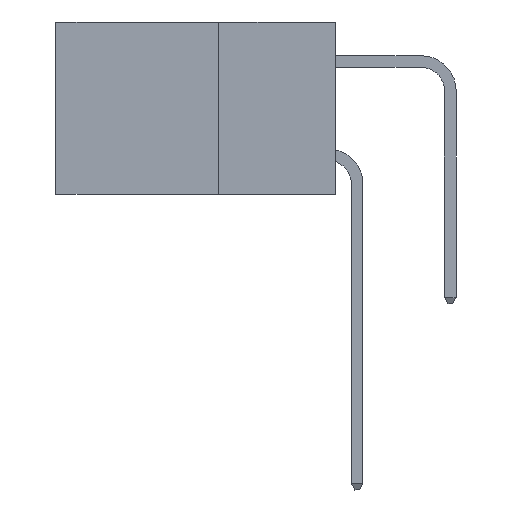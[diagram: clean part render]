
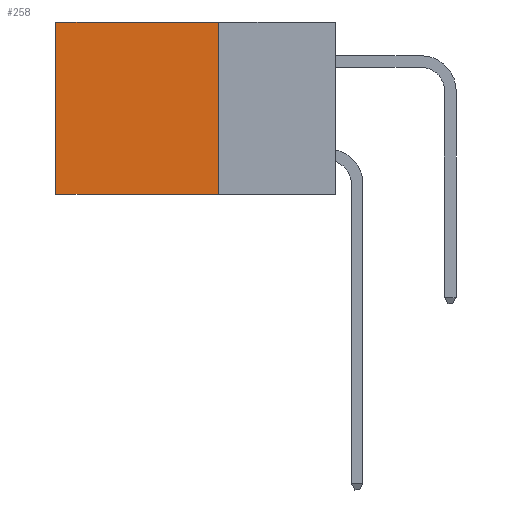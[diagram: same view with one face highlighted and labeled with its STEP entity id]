
A CAD part, left-side view. The second image highlights one B-rep face of the part: STEP entity #258.
In plain terms, the highlighted planar face has unit normal (-1, 0, 0).
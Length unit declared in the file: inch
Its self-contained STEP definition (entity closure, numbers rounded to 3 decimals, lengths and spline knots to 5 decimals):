
#137 = EDGE_CURVE ( 'NONE', #5215, #2214, #8171, .T. ) ;
#258 = ADVANCED_FACE ( 'NONE', ( #6620 ), #11562, .F. ) ;
#606 = DIRECTION ( 'NONE',  ( 0., 0., -1. ) ) ;
#1831 = CARTESIAN_POINT ( 'NONE',  ( 0.2875, 0.25, -0.37 ) ) ;
#1930 = DIRECTION ( 'NONE',  ( 0., 0., -1. ) ) ;
#1971 = CARTESIAN_POINT ( 'NONE',  ( 0.2875, 0.25, 0. ) ) ;
#2177 = LINE ( 'NONE', #2219, #7126 ) ;
#2214 = VERTEX_POINT ( 'NONE', #7448 ) ;
#2219 = CARTESIAN_POINT ( 'NONE',  ( 0.2875, 0.6, 0. ) ) ;
#3072 = VERTEX_POINT ( 'NONE', #8707 ) ;
#3559 = LINE ( 'NONE', #8544, #8493 ) ;
#3839 = CARTESIAN_POINT ( 'NONE',  ( 0.2875, 0.25, -0.37 ) ) ;
#4750 = CARTESIAN_POINT ( 'NONE',  ( 0.2875, 0.25, 0. ) ) ;
#5052 = EDGE_CURVE ( 'NONE', #3072, #2214, #2177, .T. ) ;
#5160 = DIRECTION ( 'NONE',  ( 1., 0., 0. ) ) ;
#5215 = VERTEX_POINT ( 'NONE', #3839 ) ;
#5244 = DIRECTION ( 'NONE',  ( 0., 0., -1. ) ) ;
#5316 = DIRECTION ( 'NONE',  ( 0., 1., 0. ) ) ;
#5541 = VECTOR ( 'NONE', #5316, 39.37008 ) ;
#5803 = AXIS2_PLACEMENT_3D ( 'NONE', #4750, #5160, #5244 ) ;
#5904 = ORIENTED_EDGE ( 'NONE', *, *, #5052, .T. ) ;
#6285 = VECTOR ( 'NONE', #11564, 39.37008 ) ;
#6306 = EDGE_CURVE ( 'NONE', #7110, #5215, #3559, .T. ) ;
#6620 = FACE_OUTER_BOUND ( 'NONE', #10270, .T. ) ;
#6824 = ORIENTED_EDGE ( 'NONE', *, *, #137, .F. ) ;
#7110 = VERTEX_POINT ( 'NONE', #10471 ) ;
#7126 = VECTOR ( 'NONE', #1930, 39.37008 ) ;
#7435 = ORIENTED_EDGE ( 'NONE', *, *, #6306, .F. ) ;
#7448 = CARTESIAN_POINT ( 'NONE',  ( 0.2875, 0.6, -0.37 ) ) ;
#7653 = ORIENTED_EDGE ( 'NONE', *, *, #8519, .T. ) ;
#8171 = LINE ( 'NONE', #1831, #5541 ) ;
#8493 = VECTOR ( 'NONE', #606, 39.37008 ) ;
#8519 = EDGE_CURVE ( 'NONE', #7110, #3072, #8900, .T. ) ;
#8544 = CARTESIAN_POINT ( 'NONE',  ( 0.2875, 0.25, 0. ) ) ;
#8707 = CARTESIAN_POINT ( 'NONE',  ( 0.2875, 0.6, 0. ) ) ;
#8900 = LINE ( 'NONE', #1971, #6285 ) ;
#10270 = EDGE_LOOP ( 'NONE', ( #5904, #6824, #7435, #7653 ) ) ;
#10471 = CARTESIAN_POINT ( 'NONE',  ( 0.2875, 0.25, 0. ) ) ;
#11562 = PLANE ( 'NONE',  #5803 ) ;
#11564 = DIRECTION ( 'NONE',  ( 0., 1., 0. ) ) ;
